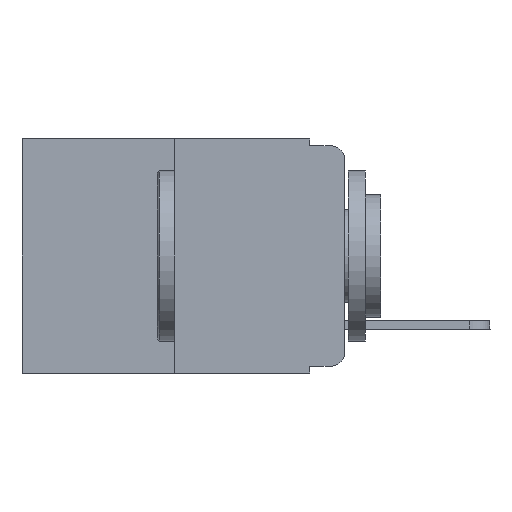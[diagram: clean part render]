
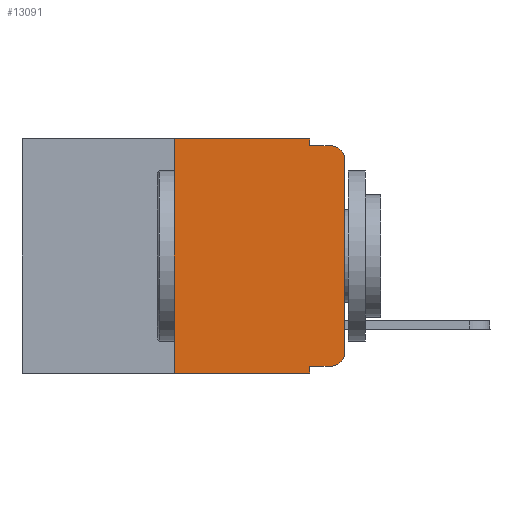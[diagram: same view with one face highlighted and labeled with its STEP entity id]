
A CAD part, left-side view. The second image highlights one B-rep face of the part: STEP entity #13091.
In plain terms, the highlighted planar face has unit normal (-1, 0, 0).
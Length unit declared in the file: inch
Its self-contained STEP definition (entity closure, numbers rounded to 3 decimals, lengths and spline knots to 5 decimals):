
#67 = CARTESIAN_POINT ( 'NONE',  ( 0., 0.051, 0. ) ) ;
#318 = CARTESIAN_POINT ( 'NONE',  ( 0., 0.051, -0.343 ) ) ;
#498 = VECTOR ( 'NONE', #7994, 39.37008 ) ;
#558 = ORIENTED_EDGE ( 'NONE', *, *, #11934, .T. ) ;
#1001 = CARTESIAN_POINT ( 'NONE',  ( 0., 0.051, 0. ) ) ;
#1014 = VERTEX_POINT ( 'NONE', #7959 ) ;
#1312 = LINE ( 'NONE', #9701, #2963 ) ;
#1450 = DIRECTION ( 'NONE',  ( 0., 0., 1. ) ) ;
#1464 = EDGE_CURVE ( 'NONE', #3843, #5326, #1578, .T. ) ;
#1543 = ORIENTED_EDGE ( 'NONE', *, *, #8018, .T. ) ;
#1567 = ORIENTED_EDGE ( 'NONE', *, *, #7319, .F. ) ;
#1578 = LINE ( 'NONE', #3723, #11612 ) ;
#1723 = CARTESIAN_POINT ( 'NONE',  ( 0., 0.02, -0.01 ) ) ;
#2053 = LINE ( 'NONE', #10793, #3630 ) ;
#2289 = DIRECTION ( 'NONE',  ( 0., 0., -1. ) ) ;
#2416 = VECTOR ( 'NONE', #1450, 39.37008 ) ;
#2532 = CARTESIAN_POINT ( 'NONE',  ( 0., 0.051, -0.01 ) ) ;
#2786 = ORIENTED_EDGE ( 'NONE', *, *, #5810, .T. ) ;
#2852 = EDGE_CURVE ( 'NONE', #6978, #3843, #2053, .T. ) ;
#2901 = CARTESIAN_POINT ( 'NONE',  ( 0., 0.473, 0. ) ) ;
#2920 = ORIENTED_EDGE ( 'NONE', *, *, #2852, .F. ) ;
#2933 = EDGE_CURVE ( 'NONE', #12851, #9186, #4178, .T. ) ;
#2963 = VECTOR ( 'NONE', #3387, 39.37008 ) ;
#2973 = DIRECTION ( 'NONE',  ( 0., 0., -1. ) ) ;
#3387 = DIRECTION ( 'NONE',  ( 0., -1., 0. ) ) ;
#3630 = VECTOR ( 'NONE', #7534, 39.37008 ) ;
#3723 = CARTESIAN_POINT ( 'NONE',  ( 0., 0.473, 0. ) ) ;
#3843 = VERTEX_POINT ( 'NONE', #6641 ) ;
#4076 = VERTEX_POINT ( 'NONE', #2532 ) ;
#4153 = DIRECTION ( 'NONE',  ( 1., 0., 0. ) ) ;
#4178 = LINE ( 'NONE', #1001, #11170 ) ;
#4848 = LINE ( 'NONE', #10851, #13040 ) ;
#4872 = ORIENTED_EDGE ( 'NONE', *, *, #10840, .T. ) ;
#4918 = DIRECTION ( 'NONE',  ( 0., -1., 0. ) ) ;
#5060 = FACE_OUTER_BOUND ( 'NONE', #9183, .T. ) ;
#5158 = DIRECTION ( 'NONE',  ( -1., 0., 0. ) ) ;
#5285 = VECTOR ( 'NONE', #2289, 39.37008 ) ;
#5320 = ORIENTED_EDGE ( 'NONE', *, *, #2933, .F. ) ;
#5326 = VERTEX_POINT ( 'NONE', #10978 ) ;
#5803 = CIRCLE ( 'NONE', #8695, 0.02 ) ;
#5810 = EDGE_CURVE ( 'NONE', #12851, #11681, #4848, .T. ) ;
#6073 = LINE ( 'NONE', #13194, #498 ) ;
#6641 = CARTESIAN_POINT ( 'NONE',  ( 0., 0.25, 0. ) ) ;
#6891 = AXIS2_PLACEMENT_3D ( 'NONE', #8057, #9048, #13267 ) ;
#6978 = VERTEX_POINT ( 'NONE', #7348 ) ;
#7319 = EDGE_CURVE ( 'NONE', #5326, #4076, #11663, .T. ) ;
#7348 = CARTESIAN_POINT ( 'NONE',  ( 0., 0.25, -0.343 ) ) ;
#7534 = DIRECTION ( 'NONE',  ( 0., 0., 1. ) ) ;
#7757 = LINE ( 'NONE', #11987, #2416 ) ;
#7959 = CARTESIAN_POINT ( 'NONE',  ( 0., 0., -0.313 ) ) ;
#7994 = DIRECTION ( 'NONE',  ( 0., -1., 0. ) ) ;
#8018 = EDGE_CURVE ( 'NONE', #1014, #11147, #7757, .T. ) ;
#8057 = CARTESIAN_POINT ( 'NONE',  ( 0., 0.02, -0.313 ) ) ;
#8071 = DIRECTION ( 'NONE',  ( 0., -1., 0. ) ) ;
#8695 = AXIS2_PLACEMENT_3D ( 'NONE', #10574, #5158, #9385 ) ;
#9038 = EDGE_CURVE ( 'NONE', #11681, #1014, #11748, .T. ) ;
#9048 = DIRECTION ( 'NONE',  ( -1., 0., 0. ) ) ;
#9106 = EDGE_CURVE ( 'NONE', #4076, #9819, #6073, .T. ) ;
#9183 = EDGE_LOOP ( 'NONE', ( #1543, #4872, #12013, #1567, #9416, #2920, #558, #5320, #2786, #9527 ) ) ;
#9186 = VERTEX_POINT ( 'NONE', #318 ) ;
#9385 = DIRECTION ( 'NONE',  ( 0., 0., -1. ) ) ;
#9416 = ORIENTED_EDGE ( 'NONE', *, *, #1464, .F. ) ;
#9527 = ORIENTED_EDGE ( 'NONE', *, *, #9038, .T. ) ;
#9701 = CARTESIAN_POINT ( 'NONE',  ( 0., 0.473, -0.343 ) ) ;
#9819 = VERTEX_POINT ( 'NONE', #1723 ) ;
#10278 = CARTESIAN_POINT ( 'NONE',  ( 0., 0., -0.03 ) ) ;
#10574 = CARTESIAN_POINT ( 'NONE',  ( 0., 0.02, -0.03 ) ) ;
#10793 = CARTESIAN_POINT ( 'NONE',  ( 0., 0.25, 0. ) ) ;
#10840 = EDGE_CURVE ( 'NONE', #11147, #9819, #5803, .T. ) ;
#10851 = CARTESIAN_POINT ( 'NONE',  ( 0., 0.051, -0.333 ) ) ;
#10978 = CARTESIAN_POINT ( 'NONE',  ( 0., 0.051, 0. ) ) ;
#11147 = VERTEX_POINT ( 'NONE', #10278 ) ;
#11170 = VECTOR ( 'NONE', #11600, 39.37008 ) ;
#11600 = DIRECTION ( 'NONE',  ( 0., 0., -1. ) ) ;
#11612 = VECTOR ( 'NONE', #8071, 39.37008 ) ;
#11663 = LINE ( 'NONE', #67, #5285 ) ;
#11681 = VERTEX_POINT ( 'NONE', #13161 ) ;
#11741 = CARTESIAN_POINT ( 'NONE',  ( 0., 0.051, -0.333 ) ) ;
#11748 = CIRCLE ( 'NONE', #6891, 0.02 ) ;
#11934 = EDGE_CURVE ( 'NONE', #6978, #9186, #1312, .T. ) ;
#11987 = CARTESIAN_POINT ( 'NONE',  ( 0., 0., 0. ) ) ;
#12013 = ORIENTED_EDGE ( 'NONE', *, *, #9106, .F. ) ;
#12554 = AXIS2_PLACEMENT_3D ( 'NONE', #2901, #4153, #2973 ) ;
#12851 = VERTEX_POINT ( 'NONE', #11741 ) ;
#13040 = VECTOR ( 'NONE', #4918, 39.37008 ) ;
#13091 = ADVANCED_FACE ( 'NONE', ( #5060 ), #13647, .F. ) ;
#13161 = CARTESIAN_POINT ( 'NONE',  ( 0., 0.02, -0.333 ) ) ;
#13194 = CARTESIAN_POINT ( 'NONE',  ( 0., 0.051, -0.01 ) ) ;
#13267 = DIRECTION ( 'NONE',  ( 0., 0., -1. ) ) ;
#13647 = PLANE ( 'NONE',  #12554 ) ;
